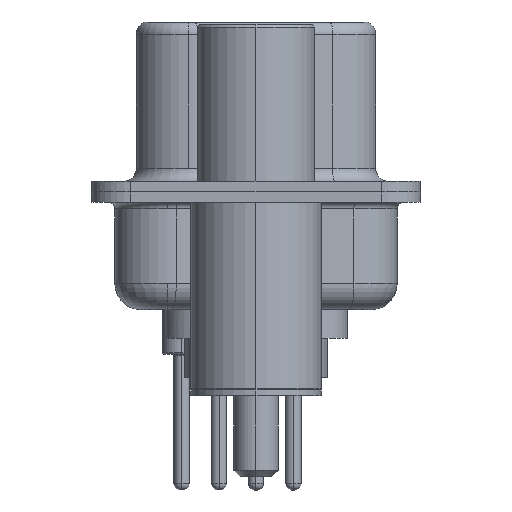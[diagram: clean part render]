
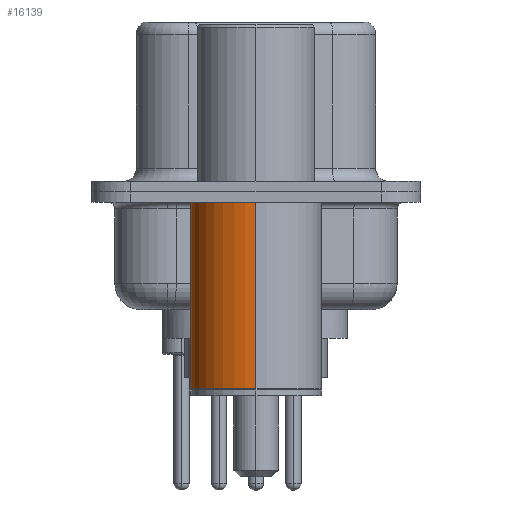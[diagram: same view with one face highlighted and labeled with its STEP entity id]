
A CAD part, left-side view. The second image highlights one B-rep face of the part: STEP entity #16139.
In plain terms, the highlighted cylindrical face has radius 2.5 mm (diameter 5 mm), a partial arc.
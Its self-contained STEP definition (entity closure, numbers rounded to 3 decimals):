
#221 = CIRCLE ( 'NONE', #4744, 2.5 ) ;
#362 = ORIENTED_EDGE ( 'NONE', *, *, #12973, .F. ) ;
#804 = DIRECTION ( 'NONE',  ( 0., 0., 1. ) ) ;
#814 = VECTOR ( 'NONE', #8055, 1000. ) ;
#1073 = CARTESIAN_POINT ( 'NONE',  ( 0., 0., 0.581 ) ) ;
#1731 = VERTEX_POINT ( 'NONE', #8732 ) ;
#2789 = CIRCLE ( 'NONE', #17933, 2.5 ) ;
#2884 = VERTEX_POINT ( 'NONE', #7111 ) ;
#4545 = ORIENTED_EDGE ( 'NONE', *, *, #6315, .F. ) ;
#4744 = AXIS2_PLACEMENT_3D ( 'NONE', #8793, #7157, #13987 ) ;
#6307 = ORIENTED_EDGE ( 'NONE', *, *, #20267, .T. ) ;
#6315 = EDGE_CURVE ( 'NONE', #2884, #1731, #10349, .T. ) ;
#6982 = CYLINDRICAL_SURFACE ( 'NONE', #15389, 2.5 ) ;
#7111 = CARTESIAN_POINT ( 'NONE',  ( 2.5, 0., -7.525 ) ) ;
#7157 = DIRECTION ( 'NONE',  ( 0., 0., 1. ) ) ;
#7614 = VECTOR ( 'NONE', #804, 1000. ) ;
#7701 = EDGE_CURVE ( 'NONE', #2884, #9534, #221, .T. ) ;
#8055 = DIRECTION ( 'NONE',  ( 0., 0., 1. ) ) ;
#8732 = CARTESIAN_POINT ( 'NONE',  ( 2.5, 0., -0.4 ) ) ;
#8793 = CARTESIAN_POINT ( 'NONE',  ( 0., 0., -7.525 ) ) ;
#9534 = VERTEX_POINT ( 'NONE', #19219 ) ;
#10349 = LINE ( 'NONE', #16158, #814 ) ;
#10615 = DIRECTION ( 'NONE',  ( 1., 0., 0. ) ) ;
#12245 = DIRECTION ( 'NONE',  ( 0., 0., 1. ) ) ;
#12973 = EDGE_CURVE ( 'NONE', #1731, #17874, #2789, .T. ) ;
#12985 = CARTESIAN_POINT ( 'NONE',  ( -2.5, 0., 0.581 ) ) ;
#13494 = CARTESIAN_POINT ( 'NONE',  ( -2.5, 0., -0.4 ) ) ;
#13987 = DIRECTION ( 'NONE',  ( 1., 0., 0. ) ) ;
#14195 = ORIENTED_EDGE ( 'NONE', *, *, #7701, .T. ) ;
#15389 = AXIS2_PLACEMENT_3D ( 'NONE', #1073, #21996, #16744 ) ;
#16128 = EDGE_LOOP ( 'NONE', ( #14195, #6307, #362, #4545 ) ) ;
#16139 = ADVANCED_FACE ( 'NONE', ( #19498 ), #6982, .T. ) ;
#16158 = CARTESIAN_POINT ( 'NONE',  ( 2.5, 0., 0.581 ) ) ;
#16744 = DIRECTION ( 'NONE',  ( 1., 0., 0. ) ) ;
#16817 = LINE ( 'NONE', #12985, #7614 ) ;
#17874 = VERTEX_POINT ( 'NONE', #13494 ) ;
#17933 = AXIS2_PLACEMENT_3D ( 'NONE', #20936, #12245, #10615 ) ;
#19219 = CARTESIAN_POINT ( 'NONE',  ( -2.5, 0., -7.525 ) ) ;
#19498 = FACE_OUTER_BOUND ( 'NONE', #16128, .T. ) ;
#20267 = EDGE_CURVE ( 'NONE', #9534, #17874, #16817, .T. ) ;
#20936 = CARTESIAN_POINT ( 'NONE',  ( 0., 0., -0.4 ) ) ;
#21996 = DIRECTION ( 'NONE',  ( 0., 0., 1. ) ) ;
